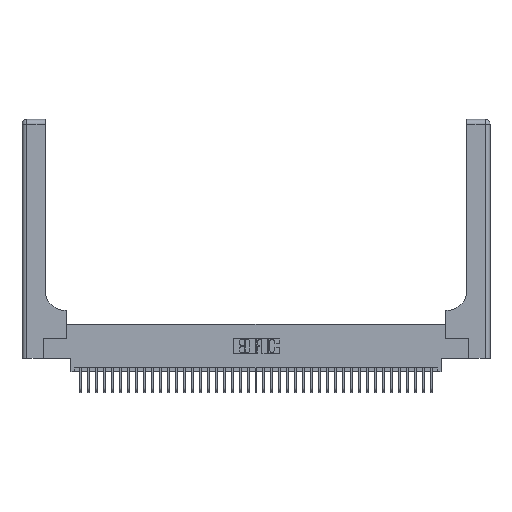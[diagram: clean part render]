
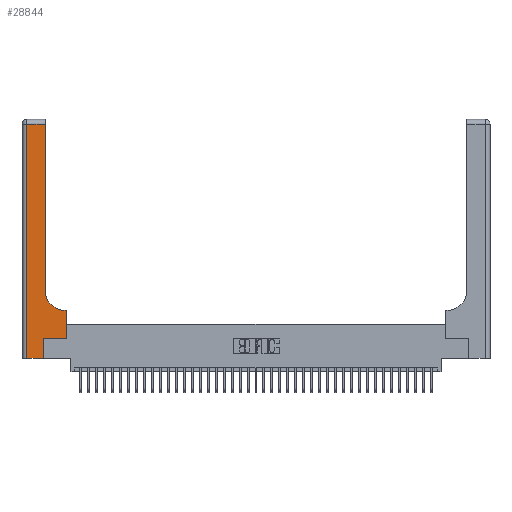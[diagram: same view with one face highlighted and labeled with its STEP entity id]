
A CAD part, top view. The second image highlights one B-rep face of the part: STEP entity #28844.
In plain terms, the highlighted planar face has unit normal (0, 0, 1).
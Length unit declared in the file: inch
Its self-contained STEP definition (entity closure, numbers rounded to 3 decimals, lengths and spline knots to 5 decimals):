
#79 = CARTESIAN_POINT ( 'NONE',  ( 0.06, 3., 0.37 ) ) ;
#1652 = VERTEX_POINT ( 'NONE', #33872 ) ;
#1836 = DIRECTION ( 'NONE',  ( 1., 0., 0. ) ) ;
#4057 = EDGE_LOOP ( 'NONE', ( #34564, #16625, #30390, #23209, #7209, #27209, #25560, #35083, #33697 ) ) ;
#4067 = LINE ( 'NONE', #26701, #27794 ) ;
#5050 = VECTOR ( 'NONE', #37456, 39.37008 ) ;
#5252 = VECTOR ( 'NONE', #10057, 39.37008 ) ;
#5361 = CARTESIAN_POINT ( 'NONE',  ( 0., 2.94, 0.37 ) ) ;
#5429 = CARTESIAN_POINT ( 'NONE',  ( 0.2915, 0.6, 0.37 ) ) ;
#5585 = CARTESIAN_POINT ( 'NONE',  ( 0.269, 0., 0.37 ) ) ;
#6286 = LINE ( 'NONE', #38390, #12866 ) ;
#6618 = CARTESIAN_POINT ( 'NONE',  ( 0.2915, 2.94, 0.37 ) ) ;
#6888 = DIRECTION ( 'NONE',  ( 0., 1., 0. ) ) ;
#6996 = CARTESIAN_POINT ( 'NONE',  ( 0., 3., 0.37 ) ) ;
#7134 = DIRECTION ( 'NONE',  ( -1., 0., 0. ) ) ;
#7209 = ORIENTED_EDGE ( 'NONE', *, *, #9598, .T. ) ;
#7930 = VECTOR ( 'NONE', #31167, 39.37008 ) ;
#8605 = DIRECTION ( 'NONE',  ( -1., 0., 0. ) ) ;
#9598 = EDGE_CURVE ( 'NONE', #13816, #31871, #35908, .T. ) ;
#9725 = AXIS2_PLACEMENT_3D ( 'NONE', #6996, #26419, #7134 ) ;
#10057 = DIRECTION ( 'NONE',  ( 0., -1., 0. ) ) ;
#10138 = CARTESIAN_POINT ( 'NONE',  ( 0.269, 0., 0.37 ) ) ;
#11260 = VECTOR ( 'NONE', #20293, 39.37008 ) ;
#11767 = CARTESIAN_POINT ( 'NONE',  ( 0.269, 0.25, 0.37 ) ) ;
#12866 = VECTOR ( 'NONE', #41603, 39.37008 ) ;
#13519 = CARTESIAN_POINT ( 'NONE',  ( 0.2915, 0.85, 0.37 ) ) ;
#13816 = VERTEX_POINT ( 'NONE', #5585 ) ;
#13836 = LINE ( 'NONE', #5361, #29914 ) ;
#13918 = DIRECTION ( 'NONE',  ( 1., 0., 0. ) ) ;
#14091 = EDGE_CURVE ( 'NONE', #14835, #1652, #22403, .T. ) ;
#14835 = VERTEX_POINT ( 'NONE', #29556 ) ;
#14902 = EDGE_CURVE ( 'NONE', #38251, #21421, #27348, .T. ) ;
#16625 = ORIENTED_EDGE ( 'NONE', *, *, #17692, .T. ) ;
#16789 = VECTOR ( 'NONE', #6888, 39.37008 ) ;
#16849 = CIRCLE ( 'NONE', #18913, 0.25 ) ;
#17055 = EDGE_CURVE ( 'NONE', #31871, #38078, #30748, .T. ) ;
#17658 = EDGE_CURVE ( 'NONE', #23291, #38251, #16849, .T. ) ;
#17692 = EDGE_CURVE ( 'NONE', #21421, #14835, #13836, .T. ) ;
#18913 = AXIS2_PLACEMENT_3D ( 'NONE', #40488, #21290, #1836 ) ;
#19148 = EDGE_CURVE ( 'NONE', #1652, #13816, #4067, .T. ) ;
#19971 = PLANE ( 'NONE',  #9725 ) ;
#20293 = DIRECTION ( 'NONE',  ( 0., 1., 0. ) ) ;
#21290 = DIRECTION ( 'NONE',  ( 0., 0., -1. ) ) ;
#21421 = VERTEX_POINT ( 'NONE', #6618 ) ;
#22403 = LINE ( 'NONE', #79, #5252 ) ;
#22481 = EDGE_CURVE ( 'NONE', #33191, #23291, #33613, .T. ) ;
#23209 = ORIENTED_EDGE ( 'NONE', *, *, #19148, .T. ) ;
#23291 = VERTEX_POINT ( 'NONE', #34905 ) ;
#25560 = ORIENTED_EDGE ( 'NONE', *, *, #36123, .T. ) ;
#26419 = DIRECTION ( 'NONE',  ( 0., 0., -1. ) ) ;
#26701 = CARTESIAN_POINT ( 'NONE',  ( 0., 0., 0.37 ) ) ;
#27209 = ORIENTED_EDGE ( 'NONE', *, *, #17055, .T. ) ;
#27348 = LINE ( 'NONE', #36306, #11260 ) ;
#27794 = VECTOR ( 'NONE', #13918, 39.37008 ) ;
#28709 = CARTESIAN_POINT ( 'NONE',  ( 0.5585, 0.25, 0.37 ) ) ;
#28844 = ADVANCED_FACE ( 'NONE', ( #28954 ), #19971, .F. ) ;
#28954 = FACE_OUTER_BOUND ( 'NONE', #4057, .T. ) ;
#29556 = CARTESIAN_POINT ( 'NONE',  ( 0.06, 2.94, 0.37 ) ) ;
#29914 = VECTOR ( 'NONE', #8605, 39.37008 ) ;
#30390 = ORIENTED_EDGE ( 'NONE', *, *, #14091, .T. ) ;
#30748 = LINE ( 'NONE', #11767, #5050 ) ;
#31167 = DIRECTION ( 'NONE',  ( -1., 0., 0. ) ) ;
#31308 = CARTESIAN_POINT ( 'NONE',  ( 0.269, 0.25, 0.37 ) ) ;
#31871 = VERTEX_POINT ( 'NONE', #31308 ) ;
#33191 = VERTEX_POINT ( 'NONE', #38586 ) ;
#33613 = LINE ( 'NONE', #5429, #7930 ) ;
#33697 = ORIENTED_EDGE ( 'NONE', *, *, #17658, .T. ) ;
#33872 = CARTESIAN_POINT ( 'NONE',  ( 0.06, 0., 0.37 ) ) ;
#34564 = ORIENTED_EDGE ( 'NONE', *, *, #14902, .T. ) ;
#34905 = CARTESIAN_POINT ( 'NONE',  ( 0.5415, 0.6, 0.37 ) ) ;
#35083 = ORIENTED_EDGE ( 'NONE', *, *, #22481, .T. ) ;
#35908 = LINE ( 'NONE', #10138, #16789 ) ;
#36123 = EDGE_CURVE ( 'NONE', #38078, #33191, #6286, .T. ) ;
#36306 = CARTESIAN_POINT ( 'NONE',  ( 0.2915, 3., 0.37 ) ) ;
#37456 = DIRECTION ( 'NONE',  ( 1., 0., 0. ) ) ;
#38078 = VERTEX_POINT ( 'NONE', #28709 ) ;
#38251 = VERTEX_POINT ( 'NONE', #13519 ) ;
#38390 = CARTESIAN_POINT ( 'NONE',  ( 0.5585, 0.25, 0.37 ) ) ;
#38586 = CARTESIAN_POINT ( 'NONE',  ( 0.5585, 0.6, 0.37 ) ) ;
#40488 = CARTESIAN_POINT ( 'NONE',  ( 0.5415, 0.85, 0.37 ) ) ;
#41603 = DIRECTION ( 'NONE',  ( 0., 1., 0. ) ) ;
